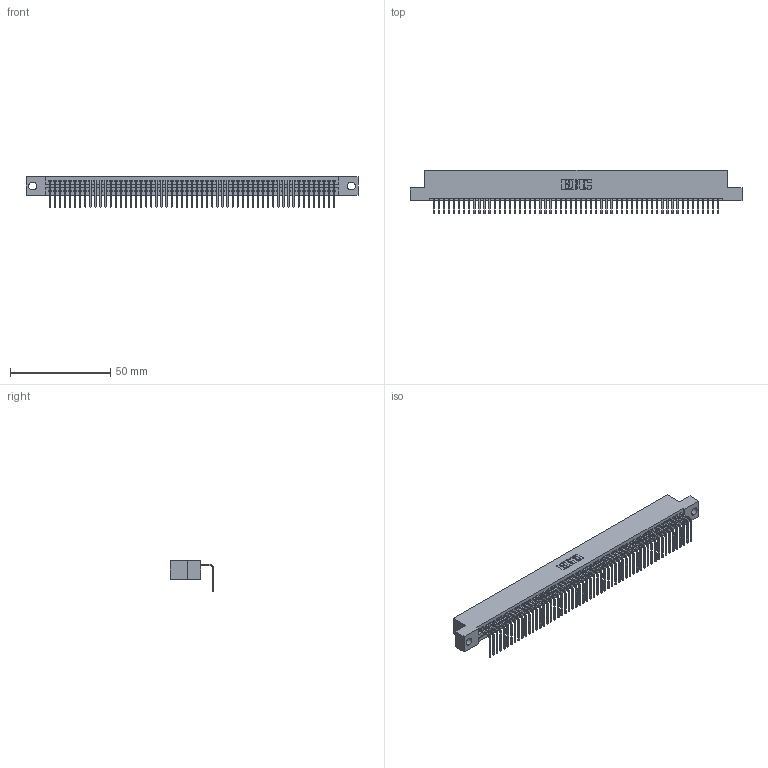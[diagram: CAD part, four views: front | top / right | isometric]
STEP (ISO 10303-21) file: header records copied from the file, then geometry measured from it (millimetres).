
FILE_DESCRIPTION (( 'STEP AP203' ), '1' );
FILE_NAME ('345-057-558-104.STEP', '2021-06-10T14:46:40', ( '' ), ( '' ), 'SwSTEP 2.0', 'SolidWorks 2020', '' );
FILE_SCHEMA (( 'CONFIG_CONTROL_DESIGN' ));
Length unit declared in the file: inch
Products named in the file (3): 345 Part_Flush Mounting Lugs - 0.156 Dia-TI; 345-292-001_558 Tail - 2; 345-057-558-104
Assembly tree (58 placements, depth 2):
  345-057-558-104
    345 Part_Flush Mounting Lugs - 0.156 Dia-TI
    345-292-001_558 Tail - 2  x57
Bounding box: 165.99 x 21.83 x 15.37 mm (x, y, z)
Volume: 15972.6 mm3; surface area: 22388.5 mm2
Topology: 58 solids, 58 shells, 3560 faces, 10751 edges, 7090 vertices
Faces by surface type: plane 2488, cylinder 1072
Entity records: 41383 total; most frequent: CARTESIAN_POINT 7177, ORIENTED_EDGE 7166, DIRECTION 6245, EDGE_CURVE 3583, LINE 3223, VECTOR 3223, VERTEX_POINT 2386, AXIS2_PLACEMENT_3D 1511
